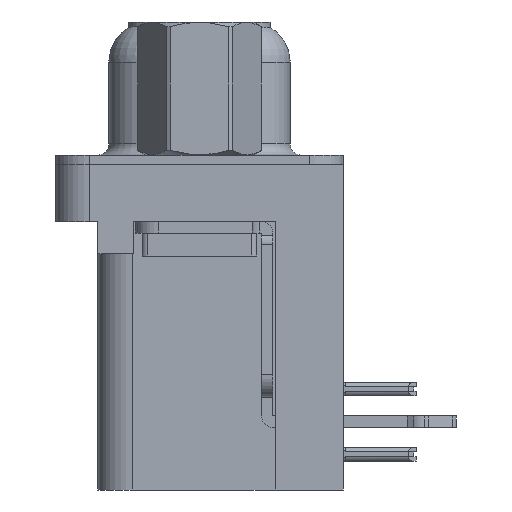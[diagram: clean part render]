
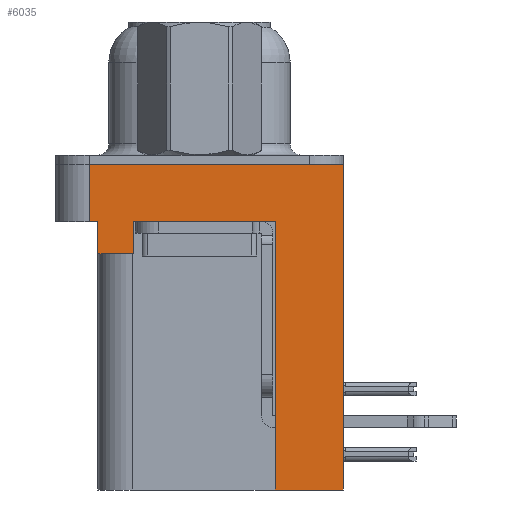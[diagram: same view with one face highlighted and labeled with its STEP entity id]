
A CAD part, left-side view. The second image highlights one B-rep face of the part: STEP entity #6035.
In plain terms, the highlighted planar face has unit normal (-1, 0, 0).
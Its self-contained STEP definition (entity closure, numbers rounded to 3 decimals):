
#641 = ORIENTED_EDGE ( 'NONE', *, *, #10080, .T. ) ;
#726 = ORIENTED_EDGE ( 'NONE', *, *, #13369, .F. ) ;
#996 = EDGE_CURVE ( 'NONE', #29286, #10130, #28472, .T. ) ;
#1002 = VERTEX_POINT ( 'NONE', #28940 ) ;
#1081 = CARTESIAN_POINT ( 'NONE',  ( -2.935, -3.295, -14.2 ) ) ;
#1210 = VECTOR ( 'NONE', #28064, 1000. ) ;
#1260 = CARTESIAN_POINT ( 'NONE',  ( -2.935, -6.275, -2.5 ) ) ;
#1546 = CARTESIAN_POINT ( 'NONE',  ( -2.935, -6.275, 0. ) ) ;
#1561 = LINE ( 'NONE', #1081, #3680 ) ;
#3680 = VECTOR ( 'NONE', #28442, 1000. ) ;
#4643 = CARTESIAN_POINT ( 'NONE',  ( -2.935, 4.775, -2.5 ) ) ;
#4957 = EDGE_CURVE ( 'NONE', #24864, #18337, #16298, .T. ) ;
#5132 = EDGE_CURVE ( 'NONE', #22559, #18337, #19368, .T. ) ;
#5574 = ORIENTED_EDGE ( 'NONE', *, *, #996, .T. ) ;
#5908 = EDGE_CURVE ( 'NONE', #23073, #10130, #26309, .T. ) ;
#6035 = ADVANCED_FACE ( 'NONE', ( #11878 ), #9612, .T. ) ;
#7367 = CARTESIAN_POINT ( 'NONE',  ( -2.935, -3.295, -14.2 ) ) ;
#8983 = VECTOR ( 'NONE', #23257, 1000. ) ;
#9234 = ORIENTED_EDGE ( 'NONE', *, *, #5132, .F. ) ;
#9612 = PLANE ( 'NONE',  #28130 ) ;
#9626 = LINE ( 'NONE', #16593, #10837 ) ;
#10052 = CARTESIAN_POINT ( 'NONE',  ( -2.935, 2.895, -3.9 ) ) ;
#10080 = EDGE_CURVE ( 'NONE', #1002, #24864, #12945, .T. ) ;
#10130 = VERTEX_POINT ( 'NONE', #13424 ) ;
#10837 = VECTOR ( 'NONE', #29214, 1000. ) ;
#11726 = DIRECTION ( 'NONE',  ( 0., 0., 1. ) ) ;
#11778 = DIRECTION ( 'NONE',  ( 0., 0., 1. ) ) ;
#11878 = FACE_OUTER_BOUND ( 'NONE', #26474, .T. ) ;
#12230 = DIRECTION ( 'NONE',  ( 0., 0., 1. ) ) ;
#12245 = ORIENTED_EDGE ( 'NONE', *, *, #26279, .F. ) ;
#12869 = VECTOR ( 'NONE', #30886, 1000. ) ;
#12945 = LINE ( 'NONE', #10052, #30455 ) ;
#13014 = VERTEX_POINT ( 'NONE', #4643 ) ;
#13035 = EDGE_CURVE ( 'NONE', #24852, #30835, #24117, .T. ) ;
#13369 = EDGE_CURVE ( 'NONE', #13014, #23073, #9626, .T. ) ;
#13424 = CARTESIAN_POINT ( 'NONE',  ( -2.935, -6.275, 0. ) ) ;
#13860 = CARTESIAN_POINT ( 'NONE',  ( -2.935, 4.775, 0. ) ) ;
#15355 = EDGE_CURVE ( 'NONE', #29286, #22559, #1561, .T. ) ;
#16298 = LINE ( 'NONE', #1260, #27059 ) ;
#16593 = CARTESIAN_POINT ( 'NONE',  ( -2.935, 4.775, -2.5 ) ) ;
#16631 = CARTESIAN_POINT ( 'NONE',  ( -2.935, -6.275, -2.5 ) ) ;
#16959 = CARTESIAN_POINT ( 'NONE',  ( -2.935, 4.425, -3.9 ) ) ;
#17061 = CARTESIAN_POINT ( 'NONE',  ( -2.935, -6.275, -2.5 ) ) ;
#17109 = ORIENTED_EDGE ( 'NONE', *, *, #5908, .F. ) ;
#17264 = VECTOR ( 'NONE', #29825, 1000. ) ;
#17544 = ORIENTED_EDGE ( 'NONE', *, *, #13035, .F. ) ;
#17745 = ORIENTED_EDGE ( 'NONE', *, *, #15355, .F. ) ;
#17753 = CARTESIAN_POINT ( 'NONE',  ( -2.935, 4.425, -2.5 ) ) ;
#18337 = VERTEX_POINT ( 'NONE', #28065 ) ;
#19368 = LINE ( 'NONE', #7367, #25015 ) ;
#20404 = DIRECTION ( 'NONE',  ( 0., 0., 1. ) ) ;
#20754 = CARTESIAN_POINT ( 'NONE',  ( -2.935, 4.425, -3.9 ) ) ;
#22559 = VERTEX_POINT ( 'NONE', #27856 ) ;
#23056 = CARTESIAN_POINT ( 'NONE',  ( -2.935, 2.895, -2.5 ) ) ;
#23073 = VERTEX_POINT ( 'NONE', #13860 ) ;
#23257 = DIRECTION ( 'NONE',  ( 0., -1., 0. ) ) ;
#23613 = DIRECTION ( 'NONE',  ( 0., -1., 0. ) ) ;
#23851 = ORIENTED_EDGE ( 'NONE', *, *, #4957, .T. ) ;
#24117 = LINE ( 'NONE', #16959, #24312 ) ;
#24312 = VECTOR ( 'NONE', #11778, 1000. ) ;
#24758 = ORIENTED_EDGE ( 'NONE', *, *, #30018, .T. ) ;
#24852 = VERTEX_POINT ( 'NONE', #20754 ) ;
#24864 = VERTEX_POINT ( 'NONE', #23056 ) ;
#25015 = VECTOR ( 'NONE', #12230, 1000. ) ;
#25151 = LINE ( 'NONE', #30461, #17264 ) ;
#25474 = LINE ( 'NONE', #30324, #1210 ) ;
#26279 = EDGE_CURVE ( 'NONE', #1002, #24852, #25474, .T. ) ;
#26309 = LINE ( 'NONE', #1546, #8983 ) ;
#26474 = EDGE_LOOP ( 'NONE', ( #17109, #726, #24758, #17544, #12245, #641, #23851, #9234, #17745, #5574 ) ) ;
#27059 = VECTOR ( 'NONE', #23613, 1000. ) ;
#27394 = CARTESIAN_POINT ( 'NONE',  ( -2.935, -6.275, -14.2 ) ) ;
#27856 = CARTESIAN_POINT ( 'NONE',  ( -2.935, -3.295, -14.2 ) ) ;
#28064 = DIRECTION ( 'NONE',  ( 0., 1., 0. ) ) ;
#28065 = CARTESIAN_POINT ( 'NONE',  ( -2.935, -3.295, -2.5 ) ) ;
#28130 = AXIS2_PLACEMENT_3D ( 'NONE', #17061, #31624, #11726 ) ;
#28442 = DIRECTION ( 'NONE',  ( 0., 1., 0. ) ) ;
#28472 = LINE ( 'NONE', #16631, #12869 ) ;
#28940 = CARTESIAN_POINT ( 'NONE',  ( -2.935, 2.895, -3.9 ) ) ;
#29214 = DIRECTION ( 'NONE',  ( 0., 0., 1. ) ) ;
#29286 = VERTEX_POINT ( 'NONE', #27394 ) ;
#29825 = DIRECTION ( 'NONE',  ( 0., -1., 0. ) ) ;
#30018 = EDGE_CURVE ( 'NONE', #13014, #30835, #25151, .T. ) ;
#30324 = CARTESIAN_POINT ( 'NONE',  ( -2.935, 4.425, -3.9 ) ) ;
#30455 = VECTOR ( 'NONE', #20404, 1000. ) ;
#30461 = CARTESIAN_POINT ( 'NONE',  ( -2.935, -6.275, -2.5 ) ) ;
#30835 = VERTEX_POINT ( 'NONE', #17753 ) ;
#30886 = DIRECTION ( 'NONE',  ( 0., 0., 1. ) ) ;
#31624 = DIRECTION ( 'NONE',  ( -1., 0., 0. ) ) ;
